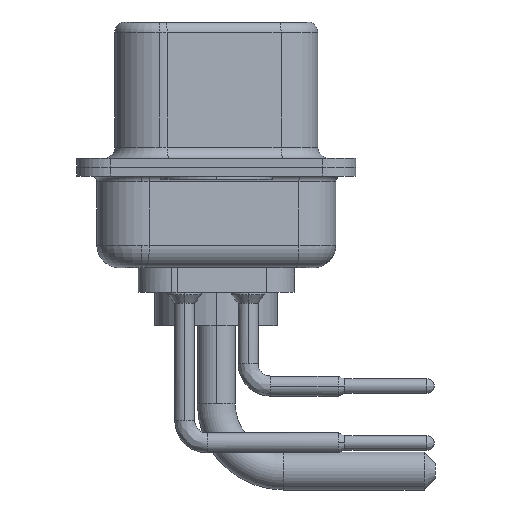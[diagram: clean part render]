
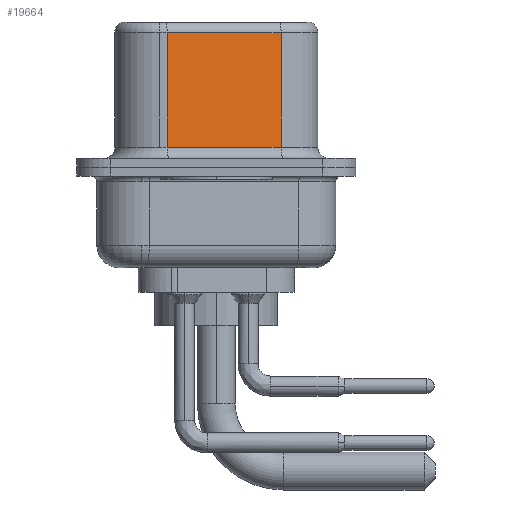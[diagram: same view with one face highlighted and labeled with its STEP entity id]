
A CAD part, left-side view. The second image highlights one B-rep face of the part: STEP entity #19664.
In plain terms, the highlighted planar face has unit normal (-0.985, -0.174, 0).
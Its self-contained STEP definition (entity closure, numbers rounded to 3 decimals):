
#1655 = LINE ( 'NONE', #6555, #3876 ) ;
#1774 = VERTEX_POINT ( 'NONE', #1910 ) ;
#1910 = CARTESIAN_POINT ( 'NONE',  ( 4.555, -2.897, 0.9 ) ) ;
#2137 = DIRECTION ( 'NONE',  ( -0.174, 0.985, 0. ) ) ;
#2536 = EDGE_CURVE ( 'NONE', #6253, #10677, #1655, .T. ) ;
#3063 = DIRECTION ( 'NONE',  ( 0., 0., -1. ) ) ;
#3876 = VECTOR ( 'NONE', #19236, 1000. ) ;
#4227 = ORIENTED_EDGE ( 'NONE', *, *, #15967, .F. ) ;
#4793 = VECTOR ( 'NONE', #8004, 1000. ) ;
#5287 = DIRECTION ( 'NONE',  ( 0.985, 0.174, 0. ) ) ;
#5504 = CARTESIAN_POINT ( 'NONE',  ( 4.555, -2.897, 6.02 ) ) ;
#5647 = EDGE_CURVE ( 'NONE', #10677, #13160, #19337, .T. ) ;
#6047 = EDGE_LOOP ( 'NONE', ( #4227, #12360, #7320, #18059 ) ) ;
#6253 = VERTEX_POINT ( 'NONE', #5504 ) ;
#6555 = CARTESIAN_POINT ( 'NONE',  ( 4.555, -2.897, 6.02 ) ) ;
#6632 = FACE_OUTER_BOUND ( 'NONE', #6047, .T. ) ;
#7320 = ORIENTED_EDGE ( 'NONE', *, *, #5647, .T. ) ;
#8004 = DIRECTION ( 'NONE',  ( 0., 0., -1. ) ) ;
#8396 = PLANE ( 'NONE',  #11496 ) ;
#9838 = DIRECTION ( 'NONE',  ( 0.174, -0.985, 0. ) ) ;
#9842 = CARTESIAN_POINT ( 'NONE',  ( 4.555, -2.897, 6.52 ) ) ;
#9973 = CARTESIAN_POINT ( 'NONE',  ( 3.655, 2.203, 6.52 ) ) ;
#10065 = VECTOR ( 'NONE', #3063, 1000. ) ;
#10677 = VERTEX_POINT ( 'NONE', #15017 ) ;
#10785 = LINE ( 'NONE', #17333, #10065 ) ;
#11496 = AXIS2_PLACEMENT_3D ( 'NONE', #9842, #5287, #2137 ) ;
#12315 = CARTESIAN_POINT ( 'NONE',  ( 3.655, 2.203, 0.9 ) ) ;
#12360 = ORIENTED_EDGE ( 'NONE', *, *, #2536, .T. ) ;
#12578 = CARTESIAN_POINT ( 'NONE',  ( 4.555, -2.897, 0.9 ) ) ;
#13065 = LINE ( 'NONE', #12578, #19069 ) ;
#13160 = VERTEX_POINT ( 'NONE', #12315 ) ;
#15017 = CARTESIAN_POINT ( 'NONE',  ( 3.655, 2.203, 6.02 ) ) ;
#15967 = EDGE_CURVE ( 'NONE', #6253, #1774, #10785, .T. ) ;
#17333 = CARTESIAN_POINT ( 'NONE',  ( 4.555, -2.897, 6.52 ) ) ;
#17986 = EDGE_CURVE ( 'NONE', #13160, #1774, #13065, .T. ) ;
#18059 = ORIENTED_EDGE ( 'NONE', *, *, #17986, .T. ) ;
#19069 = VECTOR ( 'NONE', #9838, 1000. ) ;
#19236 = DIRECTION ( 'NONE',  ( -0.174, 0.985, 0. ) ) ;
#19337 = LINE ( 'NONE', #9973, #4793 ) ;
#19664 = ADVANCED_FACE ( 'NONE', ( #6632 ), #8396, .F. ) ;
